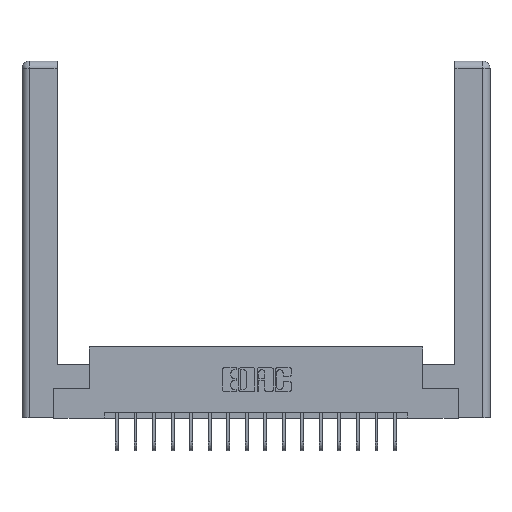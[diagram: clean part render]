
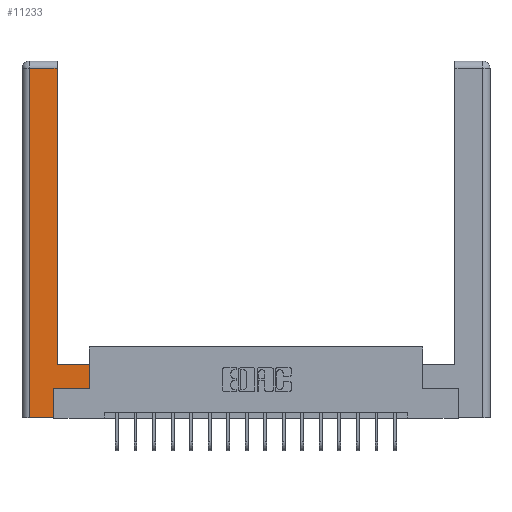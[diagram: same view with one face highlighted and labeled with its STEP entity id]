
A CAD part, top view. The second image highlights one B-rep face of the part: STEP entity #11233.
In plain terms, the highlighted planar face has unit normal (0, 0, 1).
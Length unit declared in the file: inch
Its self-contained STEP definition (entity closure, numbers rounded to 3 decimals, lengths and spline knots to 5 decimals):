
#283 = VECTOR ( 'NONE', #8579, 39.37008 ) ;
#297 = VERTEX_POINT ( 'NONE', #3895 ) ;
#461 = EDGE_CURVE ( 'NONE', #297, #2283, #9886, .T. ) ;
#934 = DIRECTION ( 'NONE',  ( 0., -1., 0. ) ) ;
#1083 = VERTEX_POINT ( 'NONE', #18367 ) ;
#1475 = EDGE_CURVE ( 'NONE', #15130, #297, #19557, .T. ) ;
#1692 = EDGE_CURVE ( 'NONE', #1083, #19866, #7853, .T. ) ;
#2283 = VERTEX_POINT ( 'NONE', #2658 ) ;
#2503 = DIRECTION ( 'NONE',  ( 0., 1., 0. ) ) ;
#2658 = CARTESIAN_POINT ( 'NONE',  ( 0.295, 0.45, 0. ) ) ;
#3139 = CARTESIAN_POINT ( 'NONE',  ( 0.565, 0.245, 0. ) ) ;
#3211 = EDGE_CURVE ( 'NONE', #9758, #1083, #10312, .T. ) ;
#3407 = ORIENTED_EDGE ( 'NONE', *, *, #1475, .T. ) ;
#3421 = PLANE ( 'NONE',  #19078 ) ;
#3470 = LINE ( 'NONE', #6745, #6146 ) ;
#3848 = VERTEX_POINT ( 'NONE', #14414 ) ;
#3895 = CARTESIAN_POINT ( 'NONE',  ( 0.565, 0.45, 0. ) ) ;
#5198 = CARTESIAN_POINT ( 'NONE',  ( 0., 0., 0. ) ) ;
#6010 = VECTOR ( 'NONE', #7822, 39.37008 ) ;
#6146 = VECTOR ( 'NONE', #934, 39.37008 ) ;
#6156 = VECTOR ( 'NONE', #18235, 39.37008 ) ;
#6201 = CARTESIAN_POINT ( 'NONE',  ( 0.0615, 2.94, 0. ) ) ;
#6308 = CARTESIAN_POINT ( 'NONE',  ( 0.295, 2.94, 0. ) ) ;
#6745 = CARTESIAN_POINT ( 'NONE',  ( 0.0615, 0., 0. ) ) ;
#6749 = DIRECTION ( 'NONE',  ( 0., 0., -1. ) ) ;
#7273 = DIRECTION ( 'NONE',  ( 0., 1., 0. ) ) ;
#7822 = DIRECTION ( 'NONE',  ( -1., 0., 0. ) ) ;
#7853 = LINE ( 'NONE', #16412, #12960 ) ;
#8579 = DIRECTION ( 'NONE',  ( 0., 1., 0. ) ) ;
#8780 = CARTESIAN_POINT ( 'NONE',  ( 0.265, 0., 0. ) ) ;
#9634 = DIRECTION ( 'NONE',  ( -1., 0., 0. ) ) ;
#9758 = VERTEX_POINT ( 'NONE', #18790 ) ;
#9840 = EDGE_CURVE ( 'NONE', #12518, #3848, #19641, .T. ) ;
#9886 = LINE ( 'NONE', #15468, #19129 ) ;
#10312 = LINE ( 'NONE', #8780, #6156 ) ;
#11122 = VECTOR ( 'NONE', #7273, 39.37008 ) ;
#11197 = ORIENTED_EDGE ( 'NONE', *, *, #19928, .T. ) ;
#11233 = ADVANCED_FACE ( 'NONE', ( #18381 ), #3421, .F. ) ;
#11342 = CARTESIAN_POINT ( 'NONE',  ( 0.565, 0.245, 0. ) ) ;
#11580 = CARTESIAN_POINT ( 'NONE',  ( 0.565, 0.45, 0. ) ) ;
#11802 = ORIENTED_EDGE ( 'NONE', *, *, #9840, .T. ) ;
#12197 = EDGE_LOOP ( 'NONE', ( #11197, #11802, #14510, #17808, #18183, #18781, #3407, #16835 ) ) ;
#12201 = EDGE_CURVE ( 'NONE', #3848, #9758, #3470, .T. ) ;
#12381 = DIRECTION ( 'NONE',  ( 1., 0., 0. ) ) ;
#12518 = VERTEX_POINT ( 'NONE', #6308 ) ;
#12960 = VECTOR ( 'NONE', #2503, 39.37008 ) ;
#13469 = CARTESIAN_POINT ( 'NONE',  ( 0.265, 0.245, 0. ) ) ;
#14414 = CARTESIAN_POINT ( 'NONE',  ( 0.0615, 2.94, 0. ) ) ;
#14510 = ORIENTED_EDGE ( 'NONE', *, *, #12201, .T. ) ;
#15130 = VERTEX_POINT ( 'NONE', #11342 ) ;
#15468 = CARTESIAN_POINT ( 'NONE',  ( 0.295, 0.45, 0. ) ) ;
#16412 = CARTESIAN_POINT ( 'NONE',  ( 0.265, 0.245, 0. ) ) ;
#16503 = LINE ( 'NONE', #3139, #16988 ) ;
#16835 = ORIENTED_EDGE ( 'NONE', *, *, #461, .T. ) ;
#16988 = VECTOR ( 'NONE', #12381, 39.37008 ) ;
#17808 = ORIENTED_EDGE ( 'NONE', *, *, #3211, .T. ) ;
#17924 = LINE ( 'NONE', #17963, #11122 ) ;
#17963 = CARTESIAN_POINT ( 'NONE',  ( 0.295, 3., 0. ) ) ;
#18183 = ORIENTED_EDGE ( 'NONE', *, *, #1692, .T. ) ;
#18235 = DIRECTION ( 'NONE',  ( 1., 0., 0. ) ) ;
#18367 = CARTESIAN_POINT ( 'NONE',  ( 0.265, 0., 0. ) ) ;
#18381 = FACE_OUTER_BOUND ( 'NONE', #12197, .T. ) ;
#18781 = ORIENTED_EDGE ( 'NONE', *, *, #19468, .T. ) ;
#18790 = CARTESIAN_POINT ( 'NONE',  ( 0.0615, 0., 0. ) ) ;
#19002 = DIRECTION ( 'NONE',  ( -1., 0., 0. ) ) ;
#19078 = AXIS2_PLACEMENT_3D ( 'NONE', #5198, #6749, #9634 ) ;
#19129 = VECTOR ( 'NONE', #19002, 39.37008 ) ;
#19468 = EDGE_CURVE ( 'NONE', #19866, #15130, #16503, .T. ) ;
#19557 = LINE ( 'NONE', #11580, #283 ) ;
#19641 = LINE ( 'NONE', #6201, #6010 ) ;
#19866 = VERTEX_POINT ( 'NONE', #13469 ) ;
#19928 = EDGE_CURVE ( 'NONE', #2283, #12518, #17924, .T. ) ;
